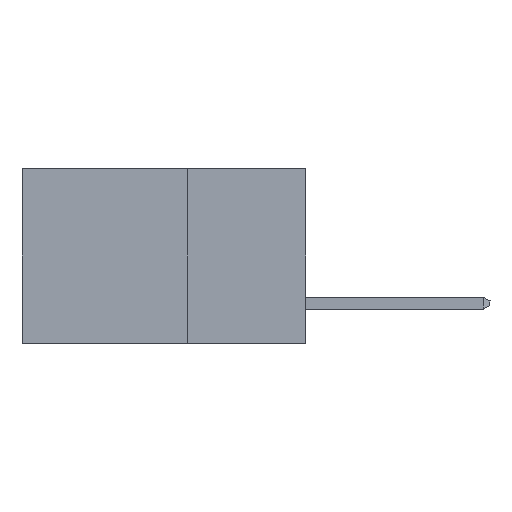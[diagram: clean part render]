
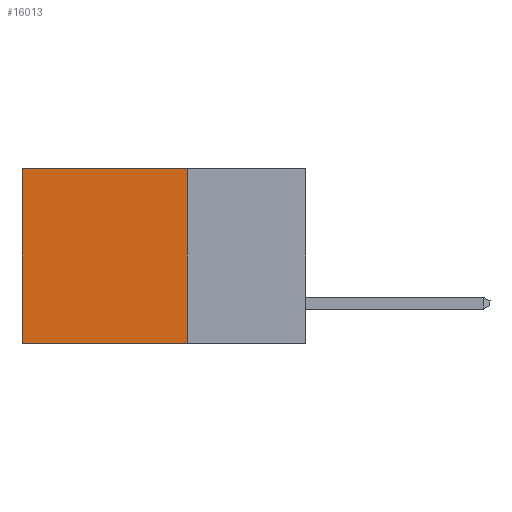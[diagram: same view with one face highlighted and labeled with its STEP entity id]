
A CAD part, left-side view. The second image highlights one B-rep face of the part: STEP entity #16013.
In plain terms, the highlighted planar face has unit normal (-1, 0, 0).
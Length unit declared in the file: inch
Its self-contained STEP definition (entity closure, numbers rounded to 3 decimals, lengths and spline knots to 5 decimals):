
#1474 = AXIS2_PLACEMENT_3D ( 'NONE', #17509, #22802, #19159 ) ;
#1727 = EDGE_CURVE ( 'NONE', #22765, #15181, #5754, .T. ) ;
#2940 = LINE ( 'NONE', #3826, #9560 ) ;
#3826 = CARTESIAN_POINT ( 'NONE',  ( 0.298, 0.6, 0. ) ) ;
#5673 = DIRECTION ( 'NONE',  ( 0., 0., -1. ) ) ;
#5754 = LINE ( 'NONE', #16732, #20976 ) ;
#5826 = CARTESIAN_POINT ( 'NONE',  ( 0.298, 0.6, -0.37 ) ) ;
#6793 = EDGE_CURVE ( 'NONE', #11235, #22765, #14735, .T. ) ;
#7668 = LINE ( 'NONE', #21881, #9412 ) ;
#8841 = CARTESIAN_POINT ( 'NONE',  ( 0.298, 0.25, 0. ) ) ;
#8862 = ORIENTED_EDGE ( 'NONE', *, *, #10053, .T. ) ;
#9367 = ORIENTED_EDGE ( 'NONE', *, *, #13424, .T. ) ;
#9412 = VECTOR ( 'NONE', #18712, 39.37008 ) ;
#9560 = VECTOR ( 'NONE', #5673, 39.37008 ) ;
#9622 = DIRECTION ( 'NONE',  ( 0., 1., 0. ) ) ;
#9809 = VERTEX_POINT ( 'NONE', #19882 ) ;
#10053 = EDGE_CURVE ( 'NONE', #9809, #15181, #2940, .T. ) ;
#11193 = EDGE_LOOP ( 'NONE', ( #8862, #22139, #17688, #9367 ) ) ;
#11235 = VERTEX_POINT ( 'NONE', #14201 ) ;
#13424 = EDGE_CURVE ( 'NONE', #11235, #9809, #7668, .T. ) ;
#13632 = PLANE ( 'NONE',  #1474 ) ;
#14201 = CARTESIAN_POINT ( 'NONE',  ( 0.298, 0.25, 0. ) ) ;
#14735 = LINE ( 'NONE', #8841, #15307 ) ;
#15181 = VERTEX_POINT ( 'NONE', #5826 ) ;
#15307 = VECTOR ( 'NONE', #18186, 39.37008 ) ;
#16013 = ADVANCED_FACE ( 'NONE', ( #17831 ), #13632, .F. ) ;
#16732 = CARTESIAN_POINT ( 'NONE',  ( 0.298, 0.25, -0.37 ) ) ;
#17509 = CARTESIAN_POINT ( 'NONE',  ( 0.298, 0.25, 0. ) ) ;
#17688 = ORIENTED_EDGE ( 'NONE', *, *, #6793, .F. ) ;
#17831 = FACE_OUTER_BOUND ( 'NONE', #11193, .T. ) ;
#18186 = DIRECTION ( 'NONE',  ( 0., 0., -1. ) ) ;
#18712 = DIRECTION ( 'NONE',  ( 0., 1., 0. ) ) ;
#19159 = DIRECTION ( 'NONE',  ( 0., 0., -1. ) ) ;
#19882 = CARTESIAN_POINT ( 'NONE',  ( 0.298, 0.6, 0. ) ) ;
#20976 = VECTOR ( 'NONE', #9622, 39.37008 ) ;
#21881 = CARTESIAN_POINT ( 'NONE',  ( 0.298, 0.25, 0. ) ) ;
#22139 = ORIENTED_EDGE ( 'NONE', *, *, #1727, .F. ) ;
#22544 = CARTESIAN_POINT ( 'NONE',  ( 0.298, 0.25, -0.37 ) ) ;
#22765 = VERTEX_POINT ( 'NONE', #22544 ) ;
#22802 = DIRECTION ( 'NONE',  ( 1., 0., 0. ) ) ;
